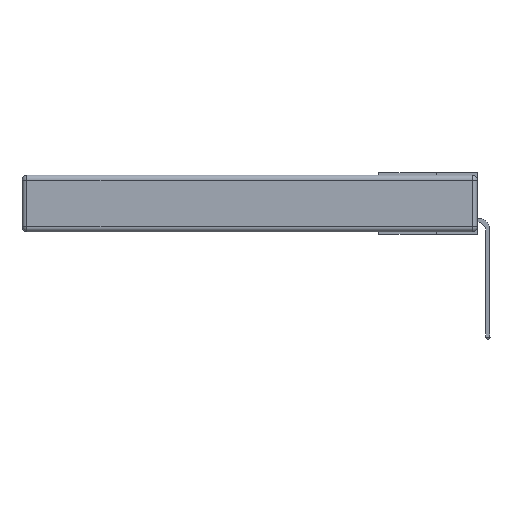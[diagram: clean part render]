
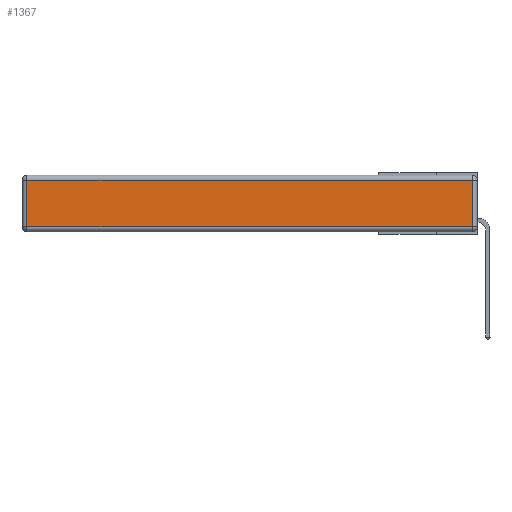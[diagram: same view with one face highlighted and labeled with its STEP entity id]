
A CAD part, left-side view. The second image highlights one B-rep face of the part: STEP entity #1367.
In plain terms, the highlighted planar face has unit normal (-1, 0, 0).
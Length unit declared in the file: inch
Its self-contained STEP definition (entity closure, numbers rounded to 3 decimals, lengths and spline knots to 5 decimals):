
#249 = CARTESIAN_POINT ( 'NONE',  ( 0., 0., -0.343 ) ) ;
#482 = ORIENTED_EDGE ( 'NONE', *, *, #10671, .T. ) ;
#701 = LINE ( 'NONE', #12489, #9185 ) ;
#1013 = VECTOR ( 'NONE', #10022, 39.37008 ) ;
#1093 = LINE ( 'NONE', #2790, #10220 ) ;
#1099 = ORIENTED_EDGE ( 'NONE', *, *, #2441, .T. ) ;
#1273 = EDGE_CURVE ( 'NONE', #9388, #7955, #6876, .T. ) ;
#1367 = ADVANCED_FACE ( 'NONE', ( #8946 ), #9574, .T. ) ;
#2103 = EDGE_LOOP ( 'NONE', ( #12856, #1099, #482, #9189 ) ) ;
#2441 = EDGE_CURVE ( 'NONE', #7955, #4385, #5202, .T. ) ;
#2755 = VERTEX_POINT ( 'NONE', #3597 ) ;
#2790 = CARTESIAN_POINT ( 'NONE',  ( 0., 2.75, -0.03 ) ) ;
#2837 = CARTESIAN_POINT ( 'NONE',  ( 0., 0.03, -0.03 ) ) ;
#3597 = CARTESIAN_POINT ( 'NONE',  ( 0., 2.72, -0.03 ) ) ;
#4385 = VERTEX_POINT ( 'NONE', #2837 ) ;
#5202 = LINE ( 'NONE', #5748, #1013 ) ;
#5370 = DIRECTION ( 'NONE',  ( 0., -1., 0. ) ) ;
#5748 = CARTESIAN_POINT ( 'NONE',  ( 0., 0.03, -0.343 ) ) ;
#6345 = CARTESIAN_POINT ( 'NONE',  ( 0., 0.03, -0.313 ) ) ;
#6413 = DIRECTION ( 'NONE',  ( 0., 0., -1. ) ) ;
#6876 = LINE ( 'NONE', #9031, #10068 ) ;
#7220 = CARTESIAN_POINT ( 'NONE',  ( 0., 2.72, -0.313 ) ) ;
#7955 = VERTEX_POINT ( 'NONE', #6345 ) ;
#8946 = FACE_OUTER_BOUND ( 'NONE', #2103, .T. ) ;
#9031 = CARTESIAN_POINT ( 'NONE',  ( 0., 0., -0.313 ) ) ;
#9185 = VECTOR ( 'NONE', #6413, 39.37008 ) ;
#9189 = ORIENTED_EDGE ( 'NONE', *, *, #12606, .T. ) ;
#9388 = VERTEX_POINT ( 'NONE', #7220 ) ;
#9487 = DIRECTION ( 'NONE',  ( -1., 0., 0. ) ) ;
#9574 = PLANE ( 'NONE',  #11737 ) ;
#10022 = DIRECTION ( 'NONE',  ( 0., 0., 1. ) ) ;
#10068 = VECTOR ( 'NONE', #5370, 39.37008 ) ;
#10220 = VECTOR ( 'NONE', #13027, 39.37008 ) ;
#10570 = DIRECTION ( 'NONE',  ( 0., 0., 1. ) ) ;
#10671 = EDGE_CURVE ( 'NONE', #4385, #2755, #1093, .T. ) ;
#11737 = AXIS2_PLACEMENT_3D ( 'NONE', #249, #9487, #10570 ) ;
#12489 = CARTESIAN_POINT ( 'NONE',  ( 0., 2.72, -0.343 ) ) ;
#12606 = EDGE_CURVE ( 'NONE', #2755, #9388, #701, .T. ) ;
#12856 = ORIENTED_EDGE ( 'NONE', *, *, #1273, .T. ) ;
#13027 = DIRECTION ( 'NONE',  ( 0., 1., 0. ) ) ;
